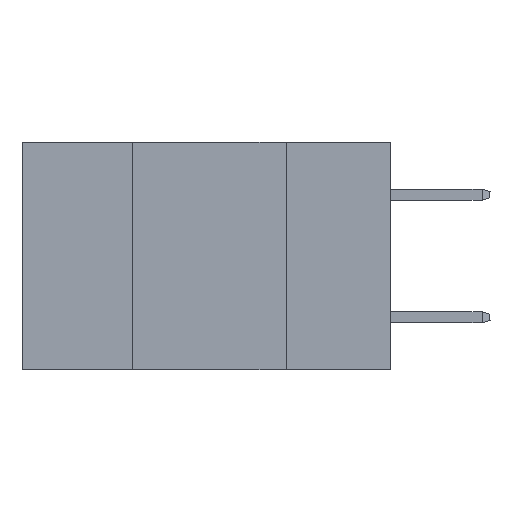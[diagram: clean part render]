
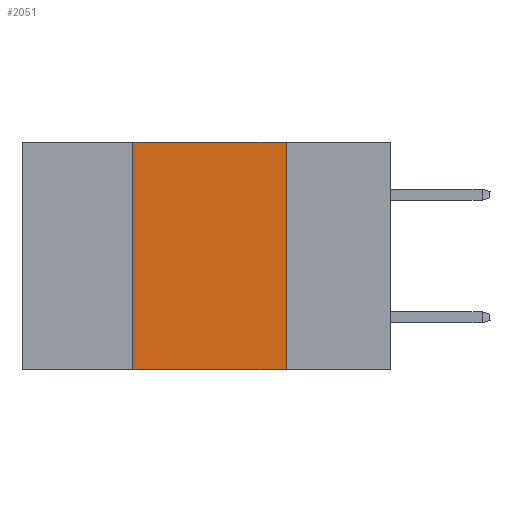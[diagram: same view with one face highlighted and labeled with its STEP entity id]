
A CAD part, left-side view. The second image highlights one B-rep face of the part: STEP entity #2051.
In plain terms, the highlighted planar face has unit normal (-1, 0, 0).
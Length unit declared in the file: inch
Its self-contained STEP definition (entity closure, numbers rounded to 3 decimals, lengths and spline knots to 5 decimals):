
#1079 = ORIENTED_EDGE ( 'NONE', *, *, #18005, .T. ) ;
#1123 = DIRECTION ( 'NONE',  ( 0., 0., 1. ) ) ;
#1978 = ORIENTED_EDGE ( 'NONE', *, *, #17432, .F. ) ;
#2051 = ADVANCED_FACE ( 'NONE', ( #17433 ), #6541, .F. ) ;
#2800 = LINE ( 'NONE', #18536, #12837 ) ;
#3976 = DIRECTION ( 'NONE',  ( 1., 0., 0. ) ) ;
#5450 = CARTESIAN_POINT ( 'NONE',  ( 0., 0.17, 0. ) ) ;
#5818 = VERTEX_POINT ( 'NONE', #8483 ) ;
#6541 = PLANE ( 'NONE',  #11475 ) ;
#6865 = DIRECTION ( 'NONE',  ( 0., 0., -1. ) ) ;
#8005 = VECTOR ( 'NONE', #10105, 39.37008 ) ;
#8330 = DIRECTION ( 'NONE',  ( 0., -1., 0. ) ) ;
#8483 = CARTESIAN_POINT ( 'NONE',  ( 0., 0.17, 0. ) ) ;
#8490 = DIRECTION ( 'NONE',  ( 0., 0., -1. ) ) ;
#8526 = VECTOR ( 'NONE', #8490, 39.37008 ) ;
#8672 = CARTESIAN_POINT ( 'NONE',  ( 0., 0.17, -0.37 ) ) ;
#8738 = LINE ( 'NONE', #5450, #8526 ) ;
#8753 = EDGE_LOOP ( 'NONE', ( #12096, #13720, #1978, #1079 ) ) ;
#10000 = VERTEX_POINT ( 'NONE', #11670 ) ;
#10052 = CARTESIAN_POINT ( 'NONE',  ( 0., 0.6, 0. ) ) ;
#10105 = DIRECTION ( 'NONE',  ( 0., -1., 0. ) ) ;
#10380 = VERTEX_POINT ( 'NONE', #8672 ) ;
#11475 = AXIS2_PLACEMENT_3D ( 'NONE', #17875, #3976, #6865 ) ;
#11670 = CARTESIAN_POINT ( 'NONE',  ( 0., 0.42, 0. ) ) ;
#11747 = EDGE_CURVE ( 'NONE', #5818, #10380, #8738, .T. ) ;
#12096 = ORIENTED_EDGE ( 'NONE', *, *, #11747, .F. ) ;
#12625 = CARTESIAN_POINT ( 'NONE',  ( 0., 0.6, -0.37 ) ) ;
#12805 = VERTEX_POINT ( 'NONE', #16489 ) ;
#12837 = VECTOR ( 'NONE', #1123, 39.37008 ) ;
#13215 = LINE ( 'NONE', #10052, #8005 ) ;
#13494 = VECTOR ( 'NONE', #8330, 39.37008 ) ;
#13720 = ORIENTED_EDGE ( 'NONE', *, *, #15840, .F. ) ;
#13972 = LINE ( 'NONE', #12625, #13494 ) ;
#15840 = EDGE_CURVE ( 'NONE', #10000, #5818, #13215, .T. ) ;
#16489 = CARTESIAN_POINT ( 'NONE',  ( 0., 0.42, -0.37 ) ) ;
#17432 = EDGE_CURVE ( 'NONE', #12805, #10000, #2800, .T. ) ;
#17433 = FACE_OUTER_BOUND ( 'NONE', #8753, .T. ) ;
#17875 = CARTESIAN_POINT ( 'NONE',  ( 0., 0.6, 0. ) ) ;
#18005 = EDGE_CURVE ( 'NONE', #12805, #10380, #13972, .T. ) ;
#18536 = CARTESIAN_POINT ( 'NONE',  ( 0., 0.42, 0. ) ) ;
